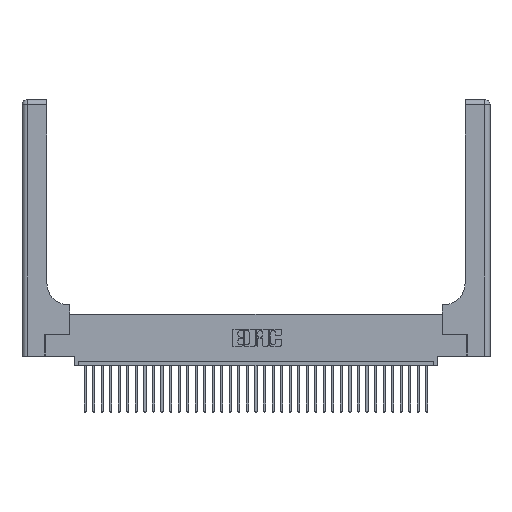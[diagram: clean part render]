
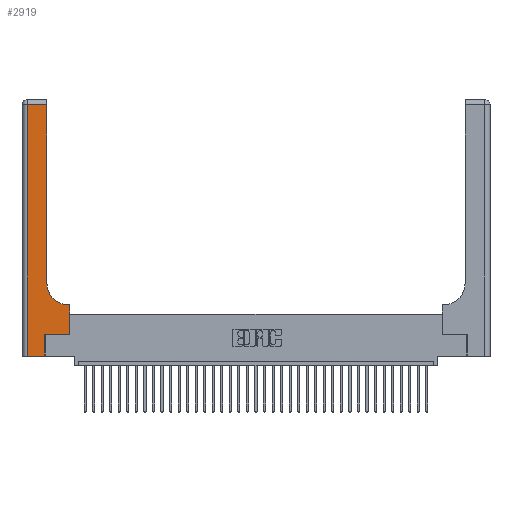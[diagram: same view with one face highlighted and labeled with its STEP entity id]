
A CAD part, top view. The second image highlights one B-rep face of the part: STEP entity #2919.
In plain terms, the highlighted planar face has unit normal (0, 0, 1).
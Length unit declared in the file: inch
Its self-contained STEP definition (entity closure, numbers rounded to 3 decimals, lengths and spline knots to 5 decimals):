
#17 = CIRCLE ( 'NONE', #31696, 0.25 ) ;
#100 = LINE ( 'NONE', #19749, #19364 ) ;
#221 = VERTEX_POINT ( 'NONE', #3907 ) ;
#390 = CARTESIAN_POINT ( 'NONE',  ( 0., 3., 0.37 ) ) ;
#850 = DIRECTION ( 'NONE',  ( 0., -1., 0. ) ) ;
#2177 = EDGE_LOOP ( 'NONE', ( #12188, #21005, #33660, #21335, #31067, #17369, #25617, #16975, #36253 ) ) ;
#2658 = EDGE_CURVE ( 'NONE', #7360, #32604, #100, .T. ) ;
#2843 = DIRECTION ( 'NONE',  ( 1., 0., 0. ) ) ;
#2919 = ADVANCED_FACE ( 'NONE', ( #36094 ), #31525, .F. ) ;
#3217 = DIRECTION ( 'NONE',  ( 0., 0., -1. ) ) ;
#3907 = CARTESIAN_POINT ( 'NONE',  ( 0.06, 2.94, 0.37 ) ) ;
#5884 = CARTESIAN_POINT ( 'NONE',  ( 0.06, 3., 0.37 ) ) ;
#6461 = CARTESIAN_POINT ( 'NONE',  ( 0.269, 0.25, 0.37 ) ) ;
#7360 = VERTEX_POINT ( 'NONE', #30675 ) ;
#8048 = CARTESIAN_POINT ( 'NONE',  ( 0.5415, 0.6, 0.37 ) ) ;
#8161 = CARTESIAN_POINT ( 'NONE',  ( 0.06, 0., 0.37 ) ) ;
#8586 = VERTEX_POINT ( 'NONE', #14134 ) ;
#8665 = VECTOR ( 'NONE', #14997, 39.37008 ) ;
#9390 = VERTEX_POINT ( 'NONE', #17875 ) ;
#9545 = CARTESIAN_POINT ( 'NONE',  ( 0.2915, 2.94, 0.37 ) ) ;
#10246 = LINE ( 'NONE', #32398, #21751 ) ;
#10976 = VERTEX_POINT ( 'NONE', #8161 ) ;
#11312 = LINE ( 'NONE', #18188, #8665 ) ;
#11825 = VERTEX_POINT ( 'NONE', #8048 ) ;
#12188 = ORIENTED_EDGE ( 'NONE', *, *, #17504, .T. ) ;
#12449 = EDGE_CURVE ( 'NONE', #9390, #7360, #17261, .T. ) ;
#14134 = CARTESIAN_POINT ( 'NONE',  ( 0.269, 0., 0.37 ) ) ;
#14412 = CARTESIAN_POINT ( 'NONE',  ( 0.5585, 0.6, 0.37 ) ) ;
#14997 = DIRECTION ( 'NONE',  ( -1., 0., 0. ) ) ;
#15059 = VECTOR ( 'NONE', #25895, 39.37008 ) ;
#15140 = VECTOR ( 'NONE', #18405, 39.37008 ) ;
#16975 = ORIENTED_EDGE ( 'NONE', *, *, #21241, .T. ) ;
#17261 = LINE ( 'NONE', #6461, #15059 ) ;
#17369 = ORIENTED_EDGE ( 'NONE', *, *, #12449, .T. ) ;
#17379 = VERTEX_POINT ( 'NONE', #9545 ) ;
#17458 = EDGE_CURVE ( 'NONE', #8586, #9390, #34903, .T. ) ;
#17504 = EDGE_CURVE ( 'NONE', #18971, #17379, #22629, .T. ) ;
#17788 = DIRECTION ( 'NONE',  ( -1., 0., 0. ) ) ;
#17875 = CARTESIAN_POINT ( 'NONE',  ( 0.269, 0.25, 0.37 ) ) ;
#18188 = CARTESIAN_POINT ( 'NONE',  ( 0., 2.94, 0.37 ) ) ;
#18405 = DIRECTION ( 'NONE',  ( 0., 1., 0. ) ) ;
#18527 = DIRECTION ( 'NONE',  ( 0., 1., 0. ) ) ;
#18971 = VERTEX_POINT ( 'NONE', #27602 ) ;
#19364 = VECTOR ( 'NONE', #24956, 39.37008 ) ;
#19749 = CARTESIAN_POINT ( 'NONE',  ( 0.5585, 0.25, 0.37 ) ) ;
#21005 = ORIENTED_EDGE ( 'NONE', *, *, #27972, .T. ) ;
#21241 = EDGE_CURVE ( 'NONE', #32604, #11825, #10246, .T. ) ;
#21335 = ORIENTED_EDGE ( 'NONE', *, *, #35634, .T. ) ;
#21751 = VECTOR ( 'NONE', #29362, 39.37008 ) ;
#21895 = DIRECTION ( 'NONE',  ( 0., 0., -1. ) ) ;
#22135 = CARTESIAN_POINT ( 'NONE',  ( 0.5415, 0.85, 0.37 ) ) ;
#22604 = CARTESIAN_POINT ( 'NONE',  ( 0., 0., 0.37 ) ) ;
#22629 = LINE ( 'NONE', #32760, #15140 ) ;
#23473 = EDGE_CURVE ( 'NONE', #221, #10976, #32951, .T. ) ;
#23792 = EDGE_CURVE ( 'NONE', #11825, #18971, #17, .T. ) ;
#24190 = CARTESIAN_POINT ( 'NONE',  ( 0.269, 0., 0.37 ) ) ;
#24431 = LINE ( 'NONE', #22604, #33177 ) ;
#24956 = DIRECTION ( 'NONE',  ( 0., 1., 0. ) ) ;
#25617 = ORIENTED_EDGE ( 'NONE', *, *, #2658, .T. ) ;
#25895 = DIRECTION ( 'NONE',  ( 1., 0., 0. ) ) ;
#26171 = VECTOR ( 'NONE', #18527, 39.37008 ) ;
#27602 = CARTESIAN_POINT ( 'NONE',  ( 0.2915, 0.85, 0.37 ) ) ;
#27972 = EDGE_CURVE ( 'NONE', #17379, #221, #11312, .T. ) ;
#29362 = DIRECTION ( 'NONE',  ( -1., 0., 0. ) ) ;
#30675 = CARTESIAN_POINT ( 'NONE',  ( 0.5585, 0.25, 0.37 ) ) ;
#31067 = ORIENTED_EDGE ( 'NONE', *, *, #17458, .T. ) ;
#31525 = PLANE ( 'NONE',  #31762 ) ;
#31696 = AXIS2_PLACEMENT_3D ( 'NONE', #22135, #21895, #33168 ) ;
#31762 = AXIS2_PLACEMENT_3D ( 'NONE', #390, #3217, #17788 ) ;
#32398 = CARTESIAN_POINT ( 'NONE',  ( 0.2915, 0.6, 0.37 ) ) ;
#32604 = VERTEX_POINT ( 'NONE', #14412 ) ;
#32760 = CARTESIAN_POINT ( 'NONE',  ( 0.2915, 3., 0.37 ) ) ;
#32951 = LINE ( 'NONE', #5884, #34720 ) ;
#33168 = DIRECTION ( 'NONE',  ( 1., 0., 0. ) ) ;
#33177 = VECTOR ( 'NONE', #2843, 39.37008 ) ;
#33660 = ORIENTED_EDGE ( 'NONE', *, *, #23473, .T. ) ;
#34720 = VECTOR ( 'NONE', #850, 39.37008 ) ;
#34903 = LINE ( 'NONE', #24190, #26171 ) ;
#35634 = EDGE_CURVE ( 'NONE', #10976, #8586, #24431, .T. ) ;
#36094 = FACE_OUTER_BOUND ( 'NONE', #2177, .T. ) ;
#36253 = ORIENTED_EDGE ( 'NONE', *, *, #23792, .T. ) ;
